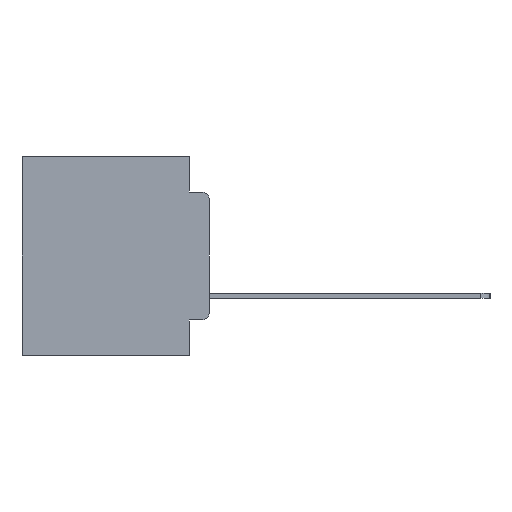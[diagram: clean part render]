
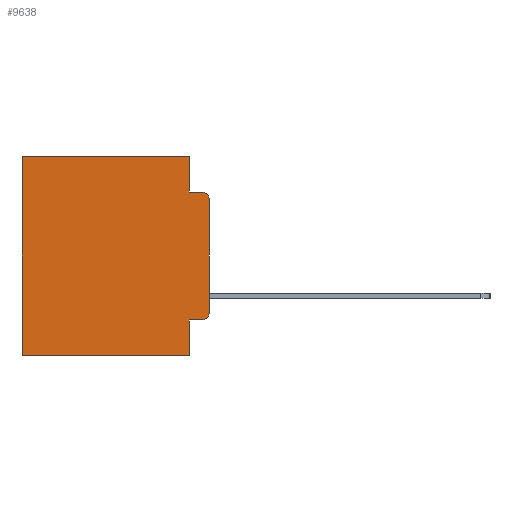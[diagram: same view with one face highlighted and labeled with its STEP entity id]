
A CAD part, left-side view. The second image highlights one B-rep face of the part: STEP entity #9638.
In plain terms, the highlighted planar face has unit normal (-1, 0, 0).
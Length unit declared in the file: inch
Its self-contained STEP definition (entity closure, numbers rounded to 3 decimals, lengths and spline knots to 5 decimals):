
#38 = LINE ( 'NONE', #18362, #5267 ) ;
#1299 = CARTESIAN_POINT ( 'NONE',  ( 0.298, 0.051, -0.0885 ) ) ;
#1595 = VECTOR ( 'NONE', #23545, 39.37008 ) ;
#1656 = VECTOR ( 'NONE', #4942, 39.37008 ) ;
#1827 = CIRCLE ( 'NONE', #10744, 0.02 ) ;
#2339 = LINE ( 'NONE', #17977, #1656 ) ;
#2450 = VECTOR ( 'NONE', #17969, 39.37008 ) ;
#3139 = LINE ( 'NONE', #17877, #2450 ) ;
#3268 = DIRECTION ( 'NONE',  ( -1., 0., 0. ) ) ;
#3635 = FACE_OUTER_BOUND ( 'NONE', #18294, .T. ) ;
#4133 = VERTEX_POINT ( 'NONE', #11169 ) ;
#4377 = CIRCLE ( 'NONE', #17085, 0.02 ) ;
#4486 = PLANE ( 'NONE',  #8152 ) ;
#4942 = DIRECTION ( 'NONE',  ( 0., 1., 0. ) ) ;
#5267 = VECTOR ( 'NONE', #7501, 39.37008 ) ;
#5665 = CARTESIAN_POINT ( 'NONE',  ( 0.298, 0.473, -0.5 ) ) ;
#5735 = VERTEX_POINT ( 'NONE', #21005 ) ;
#7019 = DIRECTION ( 'NONE',  ( 0., 0., -1. ) ) ;
#7501 = DIRECTION ( 'NONE',  ( 0., 0., -1. ) ) ;
#8152 = AXIS2_PLACEMENT_3D ( 'NONE', #8999, #23988, #11133 ) ;
#8689 = EDGE_CURVE ( 'NONE', #13365, #24461, #4377, .T. ) ;
#8946 = VERTEX_POINT ( 'NONE', #12801 ) ;
#8999 = CARTESIAN_POINT ( 'NONE',  ( 0.298, 0., 0. ) ) ;
#9638 = ADVANCED_FACE ( 'NONE', ( #3635 ), #4486, .F. ) ;
#10177 = ORIENTED_EDGE ( 'NONE', *, *, #26431, .F. ) ;
#10519 = ORIENTED_EDGE ( 'NONE', *, *, #8689, .T. ) ;
#10550 = ORIENTED_EDGE ( 'NONE', *, *, #27877, .F. ) ;
#10571 = LINE ( 'NONE', #12920, #21369 ) ;
#10599 = CARTESIAN_POINT ( 'NONE',  ( 0.298, 0., -0.1085 ) ) ;
#10744 = AXIS2_PLACEMENT_3D ( 'NONE', #25613, #12796, #27723 ) ;
#10935 = ORIENTED_EDGE ( 'NONE', *, *, #13591, .F. ) ;
#11082 = ORIENTED_EDGE ( 'NONE', *, *, #14187, .T. ) ;
#11133 = DIRECTION ( 'NONE',  ( 0., 0., -1. ) ) ;
#11169 = CARTESIAN_POINT ( 'NONE',  ( 0.298, 0.02, -0.4115 ) ) ;
#11648 = ORIENTED_EDGE ( 'NONE', *, *, #11752, .T. ) ;
#11752 = EDGE_CURVE ( 'NONE', #11840, #14779, #38, .T. ) ;
#11840 = VERTEX_POINT ( 'NONE', #12090 ) ;
#11896 = VERTEX_POINT ( 'NONE', #1299 ) ;
#11996 = ORIENTED_EDGE ( 'NONE', *, *, #20413, .F. ) ;
#12020 = ORIENTED_EDGE ( 'NONE', *, *, #20952, .F. ) ;
#12090 = CARTESIAN_POINT ( 'NONE',  ( 0.298, 0.473, 0. ) ) ;
#12095 = ORIENTED_EDGE ( 'NONE', *, *, #12290, .T. ) ;
#12290 = EDGE_CURVE ( 'NONE', #5735, #4133, #3139, .T. ) ;
#12429 = CARTESIAN_POINT ( 'NONE',  ( 0.298, 0.051, -0.5 ) ) ;
#12515 = ORIENTED_EDGE ( 'NONE', *, *, #22887, .T. ) ;
#12796 = DIRECTION ( 'NONE',  ( -1., 0., 0. ) ) ;
#12801 = CARTESIAN_POINT ( 'NONE',  ( 0.298, 0.051, 0. ) ) ;
#12920 = CARTESIAN_POINT ( 'NONE',  ( 0.298, 0., -0.5 ) ) ;
#13027 = LINE ( 'NONE', #15448, #23714 ) ;
#13348 = CARTESIAN_POINT ( 'NONE',  ( 0.298, 0.02, -0.0885 ) ) ;
#13365 = VERTEX_POINT ( 'NONE', #10599 ) ;
#13591 = EDGE_CURVE ( 'NONE', #8946, #11896, #22431, .T. ) ;
#14187 = EDGE_CURVE ( 'NONE', #8946, #11840, #2339, .T. ) ;
#14779 = VERTEX_POINT ( 'NONE', #5665 ) ;
#15128 = DIRECTION ( 'NONE',  ( 0., 1., 0. ) ) ;
#15448 = CARTESIAN_POINT ( 'NONE',  ( 0.298, 0.051, -0.0885 ) ) ;
#16142 = VECTOR ( 'NONE', #7019, 39.37008 ) ;
#16439 = CARTESIAN_POINT ( 'NONE',  ( 0.298, 0.02, -0.1085 ) ) ;
#16646 = LINE ( 'NONE', #21758, #27248 ) ;
#17085 = AXIS2_PLACEMENT_3D ( 'NONE', #16439, #3268, #18586 ) ;
#17610 = DIRECTION ( 'NONE',  ( 0., -1., 0. ) ) ;
#17877 = CARTESIAN_POINT ( 'NONE',  ( 0.298, 0.051, -0.4115 ) ) ;
#17905 = CARTESIAN_POINT ( 'NONE',  ( 0.298, 0.051, 0. ) ) ;
#17969 = DIRECTION ( 'NONE',  ( 0., -1., 0. ) ) ;
#17977 = CARTESIAN_POINT ( 'NONE',  ( 0.298, 0., 0. ) ) ;
#18294 = EDGE_LOOP ( 'NONE', ( #10177, #10519, #10550, #10935, #11082, #11648, #11996, #12020, #12095, #12515 ) ) ;
#18362 = CARTESIAN_POINT ( 'NONE',  ( 0.298, 0.473, 0. ) ) ;
#18586 = DIRECTION ( 'NONE',  ( 0., 0., -1. ) ) ;
#18861 = CARTESIAN_POINT ( 'NONE',  ( 0.298, 0., -0.3915 ) ) ;
#19180 = VERTEX_POINT ( 'NONE', #18861 ) ;
#20413 = EDGE_CURVE ( 'NONE', #26874, #14779, #10571, .T. ) ;
#20952 = EDGE_CURVE ( 'NONE', #5735, #26874, #24678, .T. ) ;
#21005 = CARTESIAN_POINT ( 'NONE',  ( 0.298, 0.051, -0.4115 ) ) ;
#21369 = VECTOR ( 'NONE', #15128, 39.37008 ) ;
#21542 = CARTESIAN_POINT ( 'NONE',  ( 0.298, 0.051, 0. ) ) ;
#21758 = CARTESIAN_POINT ( 'NONE',  ( 0.298, 0., 0. ) ) ;
#22431 = LINE ( 'NONE', #17905, #16142 ) ;
#22887 = EDGE_CURVE ( 'NONE', #4133, #19180, #1827, .T. ) ;
#23545 = DIRECTION ( 'NONE',  ( 0., 0., -1. ) ) ;
#23714 = VECTOR ( 'NONE', #17610, 39.37008 ) ;
#23861 = DIRECTION ( 'NONE',  ( 0., 0., -1. ) ) ;
#23988 = DIRECTION ( 'NONE',  ( 1., 0., 0. ) ) ;
#24461 = VERTEX_POINT ( 'NONE', #13348 ) ;
#24678 = LINE ( 'NONE', #21542, #1595 ) ;
#25613 = CARTESIAN_POINT ( 'NONE',  ( 0.298, 0.02, -0.3915 ) ) ;
#26431 = EDGE_CURVE ( 'NONE', #13365, #19180, #16646, .T. ) ;
#26874 = VERTEX_POINT ( 'NONE', #12429 ) ;
#27248 = VECTOR ( 'NONE', #23861, 39.37008 ) ;
#27723 = DIRECTION ( 'NONE',  ( 0., 0., -1. ) ) ;
#27877 = EDGE_CURVE ( 'NONE', #11896, #24461, #13027, .T. ) ;
